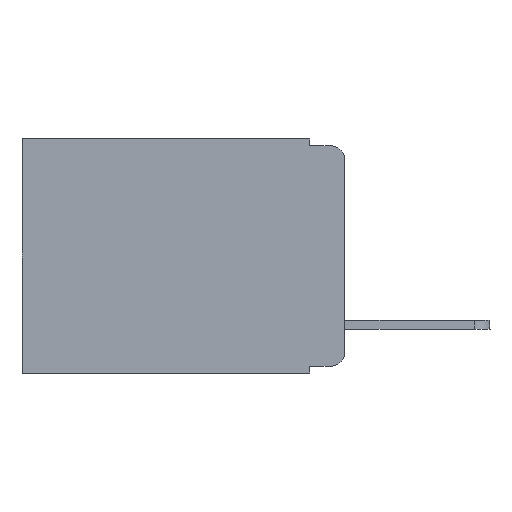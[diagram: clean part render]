
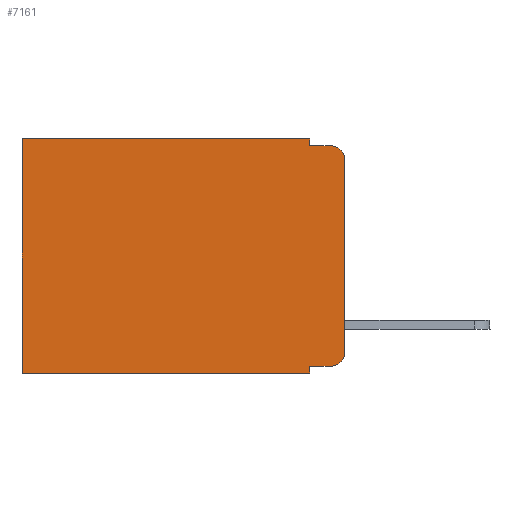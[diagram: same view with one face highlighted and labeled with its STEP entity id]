
A CAD part, left-side view. The second image highlights one B-rep face of the part: STEP entity #7161.
In plain terms, the highlighted planar face has unit normal (-1, 0, 0).
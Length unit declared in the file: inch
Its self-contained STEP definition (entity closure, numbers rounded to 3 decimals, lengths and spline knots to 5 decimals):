
#126 = VECTOR ( 'NONE', #5092, 39.37008 ) ;
#134 = DIRECTION ( 'NONE',  ( 0., 0., -1. ) ) ;
#200 = LINE ( 'NONE', #1381, #11667 ) ;
#220 = DIRECTION ( 'NONE',  ( 0., 0., -1. ) ) ;
#301 = CIRCLE ( 'NONE', #11410, 0.02 ) ;
#565 = EDGE_CURVE ( 'NONE', #11999, #8369, #1791, .T. ) ;
#676 = DIRECTION ( 'NONE',  ( 0., -1., 0. ) ) ;
#1236 = EDGE_CURVE ( 'NONE', #8088, #14396, #3688, .T. ) ;
#1381 = CARTESIAN_POINT ( 'NONE',  ( 0.298, 0.051, 0. ) ) ;
#1595 = CARTESIAN_POINT ( 'NONE',  ( 0.298, 0.051, 0. ) ) ;
#1791 = CIRCLE ( 'NONE', #4114, 0.02 ) ;
#2071 = ORIENTED_EDGE ( 'NONE', *, *, #565, .T. ) ;
#2264 = LINE ( 'NONE', #4828, #126 ) ;
#2621 = CARTESIAN_POINT ( 'NONE',  ( 0.298, 0., -0.03 ) ) ;
#3033 = LINE ( 'NONE', #7231, #15054 ) ;
#3125 = EDGE_CURVE ( 'NONE', #12770, #7787, #12673, .T. ) ;
#3688 = LINE ( 'NONE', #7890, #7905 ) ;
#3810 = CARTESIAN_POINT ( 'NONE',  ( 0.298, 0.051, -0.01 ) ) ;
#3993 = CARTESIAN_POINT ( 'NONE',  ( 0.298, 0.02, -0.01 ) ) ;
#4114 = AXIS2_PLACEMENT_3D ( 'NONE', #12426, #5457, #12610 ) ;
#4828 = CARTESIAN_POINT ( 'NONE',  ( 0.298, 0., -0.343 ) ) ;
#4863 = EDGE_CURVE ( 'NONE', #8088, #7297, #200, .T. ) ;
#4904 = ORIENTED_EDGE ( 'NONE', *, *, #3125, .F. ) ;
#4942 = DIRECTION ( 'NONE',  ( -1., 0., 0. ) ) ;
#5092 = DIRECTION ( 'NONE',  ( 0., 1., 0. ) ) ;
#5362 = LINE ( 'NONE', #13790, #14470 ) ;
#5457 = DIRECTION ( 'NONE',  ( -1., 0., 0. ) ) ;
#5540 = DIRECTION ( 'NONE',  ( 0., 0., -1. ) ) ;
#5863 = CARTESIAN_POINT ( 'NONE',  ( 0.298, 0.473, 0. ) ) ;
#5905 = EDGE_CURVE ( 'NONE', #14136, #12308, #10574, .T. ) ;
#6194 = ORIENTED_EDGE ( 'NONE', *, *, #5905, .T. ) ;
#6328 = CARTESIAN_POINT ( 'NONE',  ( 0.298, 0.051, -0.343 ) ) ;
#6507 = ORIENTED_EDGE ( 'NONE', *, *, #16212, .F. ) ;
#6530 = EDGE_LOOP ( 'NONE', ( #18063, #2071, #11470, #4904, #14160, #6194, #6507, #16224, #12401, #16888 ) ) ;
#7161 = ADVANCED_FACE ( 'NONE', ( #10103 ), #7173, .F. ) ;
#7173 = PLANE ( 'NONE',  #8743 ) ;
#7231 = CARTESIAN_POINT ( 'NONE',  ( 0.298, 0., 0. ) ) ;
#7240 = DIRECTION ( 'NONE',  ( 0., 0., -1. ) ) ;
#7297 = VERTEX_POINT ( 'NONE', #6328 ) ;
#7593 = CARTESIAN_POINT ( 'NONE',  ( 0.298, 0.02, -0.333 ) ) ;
#7787 = VERTEX_POINT ( 'NONE', #14830 ) ;
#7821 = EDGE_CURVE ( 'NONE', #14396, #12114, #301, .T. ) ;
#7890 = CARTESIAN_POINT ( 'NONE',  ( 0.298, 0.051, -0.333 ) ) ;
#7905 = VECTOR ( 'NONE', #676, 39.37008 ) ;
#8076 = CARTESIAN_POINT ( 'NONE',  ( 0.298, 0.473, -0.343 ) ) ;
#8088 = VERTEX_POINT ( 'NONE', #8765 ) ;
#8098 = LINE ( 'NONE', #3810, #14434 ) ;
#8369 = VERTEX_POINT ( 'NONE', #3993 ) ;
#8544 = VECTOR ( 'NONE', #16171, 39.37008 ) ;
#8637 = DIRECTION ( 'NONE',  ( 1., 0., 0. ) ) ;
#8743 = AXIS2_PLACEMENT_3D ( 'NONE', #14226, #8637, #220 ) ;
#8765 = CARTESIAN_POINT ( 'NONE',  ( 0.298, 0.051, -0.333 ) ) ;
#9612 = CARTESIAN_POINT ( 'NONE',  ( 0.298, 0.051, 0. ) ) ;
#10103 = FACE_OUTER_BOUND ( 'NONE', #6530, .T. ) ;
#10574 = LINE ( 'NONE', #16263, #8544 ) ;
#11410 = AXIS2_PLACEMENT_3D ( 'NONE', #11993, #4942, #14751 ) ;
#11470 = ORIENTED_EDGE ( 'NONE', *, *, #13063, .F. ) ;
#11667 = VECTOR ( 'NONE', #7240, 39.37008 ) ;
#11758 = CARTESIAN_POINT ( 'NONE',  ( 0.298, 0., -0.313 ) ) ;
#11993 = CARTESIAN_POINT ( 'NONE',  ( 0.298, 0.02, -0.313 ) ) ;
#11999 = VERTEX_POINT ( 'NONE', #2621 ) ;
#12114 = VERTEX_POINT ( 'NONE', #11758 ) ;
#12225 = DIRECTION ( 'NONE',  ( 0., -1., 0. ) ) ;
#12308 = VERTEX_POINT ( 'NONE', #8076 ) ;
#12401 = ORIENTED_EDGE ( 'NONE', *, *, #1236, .T. ) ;
#12426 = CARTESIAN_POINT ( 'NONE',  ( 0.298, 0.02, -0.03 ) ) ;
#12610 = DIRECTION ( 'NONE',  ( 0., 0., -1. ) ) ;
#12673 = LINE ( 'NONE', #1595, #14035 ) ;
#12770 = VERTEX_POINT ( 'NONE', #9612 ) ;
#12824 = DIRECTION ( 'NONE',  ( 0., 1., 0. ) ) ;
#13063 = EDGE_CURVE ( 'NONE', #7787, #8369, #8098, .T. ) ;
#13790 = CARTESIAN_POINT ( 'NONE',  ( 0.298, 0., 0. ) ) ;
#14035 = VECTOR ( 'NONE', #134, 39.37008 ) ;
#14136 = VERTEX_POINT ( 'NONE', #5863 ) ;
#14160 = ORIENTED_EDGE ( 'NONE', *, *, #14215, .T. ) ;
#14215 = EDGE_CURVE ( 'NONE', #12770, #14136, #3033, .T. ) ;
#14226 = CARTESIAN_POINT ( 'NONE',  ( 0.298, 0., 0. ) ) ;
#14396 = VERTEX_POINT ( 'NONE', #7593 ) ;
#14434 = VECTOR ( 'NONE', #12225, 39.37008 ) ;
#14470 = VECTOR ( 'NONE', #5540, 39.37008 ) ;
#14751 = DIRECTION ( 'NONE',  ( 0., 0., -1. ) ) ;
#14830 = CARTESIAN_POINT ( 'NONE',  ( 0.298, 0.051, -0.01 ) ) ;
#15054 = VECTOR ( 'NONE', #12824, 39.37008 ) ;
#16171 = DIRECTION ( 'NONE',  ( 0., 0., -1. ) ) ;
#16212 = EDGE_CURVE ( 'NONE', #7297, #12308, #2264, .T. ) ;
#16224 = ORIENTED_EDGE ( 'NONE', *, *, #4863, .F. ) ;
#16263 = CARTESIAN_POINT ( 'NONE',  ( 0.298, 0.473, 0. ) ) ;
#16286 = EDGE_CURVE ( 'NONE', #11999, #12114, #5362, .T. ) ;
#16888 = ORIENTED_EDGE ( 'NONE', *, *, #7821, .T. ) ;
#18063 = ORIENTED_EDGE ( 'NONE', *, *, #16286, .F. ) ;
